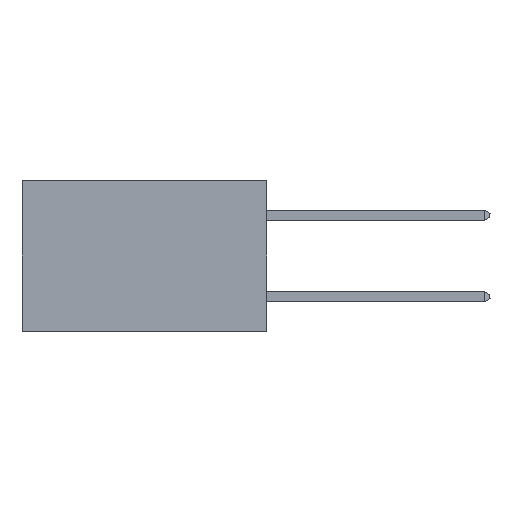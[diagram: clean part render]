
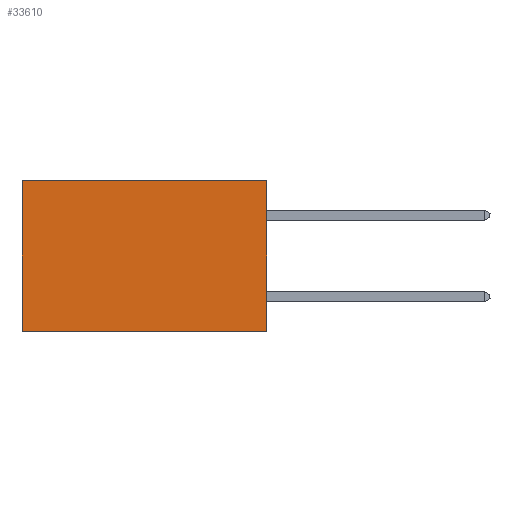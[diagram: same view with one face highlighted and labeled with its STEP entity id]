
A CAD part, left-side view. The second image highlights one B-rep face of the part: STEP entity #33610.
In plain terms, the highlighted planar face has unit normal (-1, 0, 0).
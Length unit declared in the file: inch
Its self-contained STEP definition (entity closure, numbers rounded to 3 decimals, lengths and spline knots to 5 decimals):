
#340 = ORIENTED_EDGE ( 'NONE', *, *, #38083, .F. ) ;
#891 = DIRECTION ( 'NONE',  ( 0., 0., -1. ) ) ;
#1548 = ORIENTED_EDGE ( 'NONE', *, *, #36680, .F. ) ;
#3661 = AXIS2_PLACEMENT_3D ( 'NONE', #18326, #7856, #891 ) ;
#3980 = ORIENTED_EDGE ( 'NONE', *, *, #24140, .T. ) ;
#5652 = VECTOR ( 'NONE', #23130, 39.37008 ) ;
#7856 = DIRECTION ( 'NONE',  ( 1., 0., 0. ) ) ;
#8510 = LINE ( 'NONE', #37662, #41261 ) ;
#8633 = ORIENTED_EDGE ( 'NONE', *, *, #21386, .T. ) ;
#11266 = VERTEX_POINT ( 'NONE', #17516 ) ;
#11535 = PLANE ( 'NONE',  #3661 ) ;
#11586 = FACE_OUTER_BOUND ( 'NONE', #22264, .T. ) ;
#15124 = DIRECTION ( 'NONE',  ( 0., 1., 0. ) ) ;
#17516 = CARTESIAN_POINT ( 'NONE',  ( 0.2875, 0.6, 0. ) ) ;
#18326 = CARTESIAN_POINT ( 'NONE',  ( 0.2875, 0., 0. ) ) ;
#18640 = VERTEX_POINT ( 'NONE', #37496 ) ;
#18772 = DIRECTION ( 'NONE',  ( 0., 0., -1. ) ) ;
#19006 = CARTESIAN_POINT ( 'NONE',  ( 0.2875, 0., 0. ) ) ;
#20159 = VERTEX_POINT ( 'NONE', #30980 ) ;
#20189 = LINE ( 'NONE', #19006, #30771 ) ;
#21386 = EDGE_CURVE ( 'NONE', #18640, #11266, #20189, .T. ) ;
#21669 = VECTOR ( 'NONE', #18772, 39.37008 ) ;
#22264 = EDGE_LOOP ( 'NONE', ( #3980, #340, #1548, #8633 ) ) ;
#23130 = DIRECTION ( 'NONE',  ( 0., 1., 0. ) ) ;
#24140 = EDGE_CURVE ( 'NONE', #11266, #30481, #8510, .T. ) ;
#24309 = LINE ( 'NONE', #32708, #21669 ) ;
#26511 = CARTESIAN_POINT ( 'NONE',  ( 0.2875, 0., -0.37 ) ) ;
#26900 = CARTESIAN_POINT ( 'NONE',  ( 0.2875, 0.6, -0.37 ) ) ;
#27311 = LINE ( 'NONE', #26511, #5652 ) ;
#30481 = VERTEX_POINT ( 'NONE', #26900 ) ;
#30771 = VECTOR ( 'NONE', #15124, 39.37008 ) ;
#30980 = CARTESIAN_POINT ( 'NONE',  ( 0.2875, 0., -0.37 ) ) ;
#32708 = CARTESIAN_POINT ( 'NONE',  ( 0.2875, 0., 0. ) ) ;
#33610 = ADVANCED_FACE ( 'NONE', ( #11586 ), #11535, .F. ) ;
#36680 = EDGE_CURVE ( 'NONE', #18640, #20159, #24309, .T. ) ;
#37496 = CARTESIAN_POINT ( 'NONE',  ( 0.2875, 0., 0. ) ) ;
#37537 = DIRECTION ( 'NONE',  ( 0., 0., -1. ) ) ;
#37662 = CARTESIAN_POINT ( 'NONE',  ( 0.2875, 0.6, 0. ) ) ;
#38083 = EDGE_CURVE ( 'NONE', #20159, #30481, #27311, .T. ) ;
#41261 = VECTOR ( 'NONE', #37537, 39.37008 ) ;
